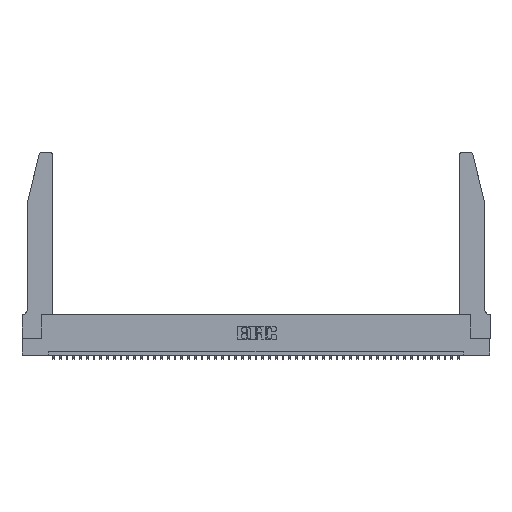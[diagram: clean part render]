
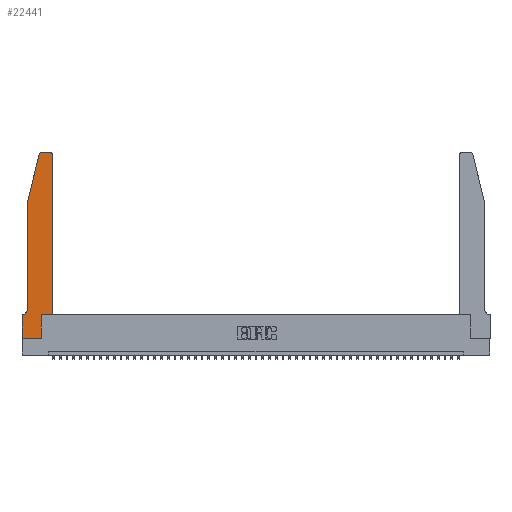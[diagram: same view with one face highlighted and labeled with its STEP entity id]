
A CAD part, top view. The second image highlights one B-rep face of the part: STEP entity #22441.
In plain terms, the highlighted planar face has unit normal (0, 0, 1).
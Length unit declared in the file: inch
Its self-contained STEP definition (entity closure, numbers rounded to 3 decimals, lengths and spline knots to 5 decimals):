
#888 = CARTESIAN_POINT ( 'NONE',  ( 0.284, 2.72, 0.37 ) ) ;
#1175 = EDGE_CURVE ( 'NONE', #20251, #20130, #47369, .T. ) ;
#1424 = CARTESIAN_POINT ( 'NONE',  ( 0.25487, 2.72718, 0.37 ) ) ;
#2176 = CARTESIAN_POINT ( 'NONE',  ( 0.4205, 2.75, 0.37 ) ) ;
#2467 = DIRECTION ( 'NONE',  ( 0., 0., -1. ) ) ;
#2583 = ORIENTED_EDGE ( 'NONE', *, *, #41564, .T. ) ;
#3452 = VERTEX_POINT ( 'NONE', #16104 ) ;
#3637 = EDGE_LOOP ( 'NONE', ( #12879, #6834, #15488, #10900, #33088, #27294, #2583, #42408, #19383, #10846, #44441, #9674 ) ) ;
#3823 = CARTESIAN_POINT ( 'NONE',  ( 0.4505, 0.35, 0.37 ) ) ;
#4202 = VECTOR ( 'NONE', #19334, 39.37008 ) ;
#4377 = CARTESIAN_POINT ( 'NONE',  ( 0., 0.35, 0.37 ) ) ;
#4639 = DIRECTION ( 'NONE',  ( 0., 0., 1. ) ) ;
#5919 = EDGE_CURVE ( 'NONE', #20130, #3452, #37285, .T. ) ;
#6834 = ORIENTED_EDGE ( 'NONE', *, *, #26370, .T. ) ;
#6891 = VERTEX_POINT ( 'NONE', #4377 ) ;
#7034 = DIRECTION ( 'NONE',  ( 0., 0., 1. ) ) ;
#7795 = DIRECTION ( 'NONE',  ( -0.239, -0.971, 0. ) ) ;
#8028 = DIRECTION ( 'NONE',  ( 0., 1., 0. ) ) ;
#8306 = CARTESIAN_POINT ( 'NONE',  ( 0., 0., 0.37 ) ) ;
#8503 = FACE_OUTER_BOUND ( 'NONE', #3637, .T. ) ;
#8516 = VECTOR ( 'NONE', #7795, 39.37008 ) ;
#9674 = ORIENTED_EDGE ( 'NONE', *, *, #22299, .T. ) ;
#10075 = AXIS2_PLACEMENT_3D ( 'NONE', #888, #4639, #22756 ) ;
#10118 = DIRECTION ( 'NONE',  ( 1., 0., 0. ) ) ;
#10243 = VERTEX_POINT ( 'NONE', #34346 ) ;
#10590 = CARTESIAN_POINT ( 'NONE',  ( 0.4505, 0.35, 0.37 ) ) ;
#10716 = VECTOR ( 'NONE', #13665, 39.37008 ) ;
#10846 = ORIENTED_EDGE ( 'NONE', *, *, #1175, .T. ) ;
#10900 = ORIENTED_EDGE ( 'NONE', *, *, #29749, .T. ) ;
#12879 = ORIENTED_EDGE ( 'NONE', *, *, #35549, .T. ) ;
#13095 = VERTEX_POINT ( 'NONE', #27475 ) ;
#13665 = DIRECTION ( 'NONE',  ( 0., -1., 0. ) ) ;
#13673 = VECTOR ( 'NONE', #8028, 39.37008 ) ;
#13694 = CARTESIAN_POINT ( 'NONE',  ( 0.0055, 0.42, 0.37 ) ) ;
#14816 = LINE ( 'NONE', #39067, #10716 ) ;
#15164 = CARTESIAN_POINT ( 'NONE',  ( 0.0755, 2., 0.37 ) ) ;
#15327 = LINE ( 'NONE', #27304, #42169 ) ;
#15488 = ORIENTED_EDGE ( 'NONE', *, *, #44695, .T. ) ;
#15513 = CARTESIAN_POINT ( 'NONE',  ( 0.2865, 0.35, 0.37 ) ) ;
#16083 = CARTESIAN_POINT ( 'NONE',  ( 0.2865, 0., 0.37 ) ) ;
#16104 = CARTESIAN_POINT ( 'NONE',  ( 0.4505, 2.72, 0.37 ) ) ;
#17557 = CARTESIAN_POINT ( 'NONE',  ( 0., 0.35, 0.37 ) ) ;
#19334 = DIRECTION ( 'NONE',  ( 0., -1., 0. ) ) ;
#19383 = ORIENTED_EDGE ( 'NONE', *, *, #28497, .T. ) ;
#20130 = VERTEX_POINT ( 'NONE', #3823 ) ;
#20251 = VERTEX_POINT ( 'NONE', #43205 ) ;
#20306 = DIRECTION ( 'NONE',  ( -1., 0., 0. ) ) ;
#20467 = CIRCLE ( 'NONE', #35473, 0.07 ) ;
#20495 = AXIS2_PLACEMENT_3D ( 'NONE', #42250, #36493, #44182 ) ;
#20784 = DIRECTION ( 'NONE',  ( 1., 0., 0. ) ) ;
#21115 = VECTOR ( 'NONE', #33774, 39.37008 ) ;
#21683 = EDGE_CURVE ( 'NONE', #13095, #44788, #33016, .T. ) ;
#22299 = EDGE_CURVE ( 'NONE', #3452, #41234, #39981, .T. ) ;
#22441 = ADVANCED_FACE ( 'NONE', ( #8503 ), #44295, .T. ) ;
#22756 = DIRECTION ( 'NONE',  ( 1., 0., 0. ) ) ;
#23231 = VERTEX_POINT ( 'NONE', #15164 ) ;
#24888 = DIRECTION ( 'NONE',  ( -1., 0., 0. ) ) ;
#26370 = EDGE_CURVE ( 'NONE', #10243, #32282, #32399, .T. ) ;
#26990 = CARTESIAN_POINT ( 'NONE',  ( 0.0055, 0.35, 0.37 ) ) ;
#27294 = ORIENTED_EDGE ( 'NONE', *, *, #44986, .T. ) ;
#27304 = CARTESIAN_POINT ( 'NONE',  ( 0.2605, 2.75, 0.37 ) ) ;
#27475 = CARTESIAN_POINT ( 'NONE',  ( 0., 0., 0.37 ) ) ;
#28497 = EDGE_CURVE ( 'NONE', #44788, #20251, #29864, .T. ) ;
#29749 = EDGE_CURVE ( 'NONE', #23231, #44315, #14816, .T. ) ;
#29864 = LINE ( 'NONE', #15513, #13673 ) ;
#31601 = CARTESIAN_POINT ( 'NONE',  ( 0.0755, 0.42, 0.37 ) ) ;
#31698 = CARTESIAN_POINT ( 'NONE',  ( 0., 0., 0.37 ) ) ;
#32230 = CARTESIAN_POINT ( 'NONE',  ( 0.4505, 0.35, 0.37 ) ) ;
#32282 = VERTEX_POINT ( 'NONE', #1424 ) ;
#32399 = CIRCLE ( 'NONE', #10075, 0.03 ) ;
#32491 = VERTEX_POINT ( 'NONE', #26990 ) ;
#33016 = LINE ( 'NONE', #31698, #36569 ) ;
#33088 = ORIENTED_EDGE ( 'NONE', *, *, #41860, .T. ) ;
#33774 = DIRECTION ( 'NONE',  ( 1., 0., 0. ) ) ;
#33883 = AXIS2_PLACEMENT_3D ( 'NONE', #17557, #7034, #10118 ) ;
#34346 = CARTESIAN_POINT ( 'NONE',  ( 0.284, 2.75, 0.37 ) ) ;
#35473 = AXIS2_PLACEMENT_3D ( 'NONE', #13694, #2467, #24888 ) ;
#35549 = EDGE_CURVE ( 'NONE', #41234, #10243, #15327, .T. ) ;
#35650 = CARTESIAN_POINT ( 'NONE',  ( 0.0755, 0.35, 0.37 ) ) ;
#35958 = LINE ( 'NONE', #35650, #39473 ) ;
#36493 = DIRECTION ( 'NONE',  ( 0., 0., 1. ) ) ;
#36569 = VECTOR ( 'NONE', #20784, 39.37008 ) ;
#37285 = LINE ( 'NONE', #32230, #41333 ) ;
#37337 = LINE ( 'NONE', #8306, #4202 ) ;
#39067 = CARTESIAN_POINT ( 'NONE',  ( 0.0755, 2., 0.37 ) ) ;
#39473 = VECTOR ( 'NONE', #20306, 39.37008 ) ;
#39593 = DIRECTION ( 'NONE',  ( 0., 1., 0. ) ) ;
#39981 = CIRCLE ( 'NONE', #20495, 0.03 ) ;
#41234 = VERTEX_POINT ( 'NONE', #2176 ) ;
#41333 = VECTOR ( 'NONE', #39593, 39.37008 ) ;
#41564 = EDGE_CURVE ( 'NONE', #6891, #13095, #37337, .T. ) ;
#41651 = CARTESIAN_POINT ( 'NONE',  ( 0.0755, 2., 0.37 ) ) ;
#41860 = EDGE_CURVE ( 'NONE', #44315, #32491, #20467, .T. ) ;
#42169 = VECTOR ( 'NONE', #42672, 39.37008 ) ;
#42250 = CARTESIAN_POINT ( 'NONE',  ( 0.4205, 2.72, 0.37 ) ) ;
#42408 = ORIENTED_EDGE ( 'NONE', *, *, #21683, .T. ) ;
#42672 = DIRECTION ( 'NONE',  ( -1., 0., 0. ) ) ;
#43205 = CARTESIAN_POINT ( 'NONE',  ( 0.2865, 0.35, 0.37 ) ) ;
#44182 = DIRECTION ( 'NONE',  ( 1., 0., 0. ) ) ;
#44295 = PLANE ( 'NONE',  #33883 ) ;
#44315 = VERTEX_POINT ( 'NONE', #31601 ) ;
#44441 = ORIENTED_EDGE ( 'NONE', *, *, #5919, .T. ) ;
#44695 = EDGE_CURVE ( 'NONE', #32282, #23231, #45218, .T. ) ;
#44788 = VERTEX_POINT ( 'NONE', #16083 ) ;
#44986 = EDGE_CURVE ( 'NONE', #32491, #6891, #35958, .T. ) ;
#45218 = LINE ( 'NONE', #41651, #8516 ) ;
#47369 = LINE ( 'NONE', #10590, #21115 ) ;
